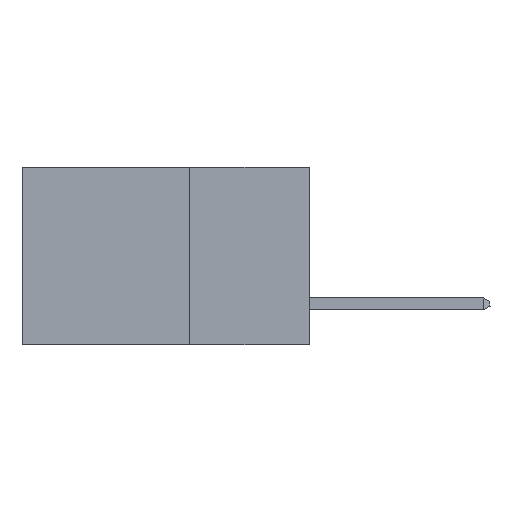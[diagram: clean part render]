
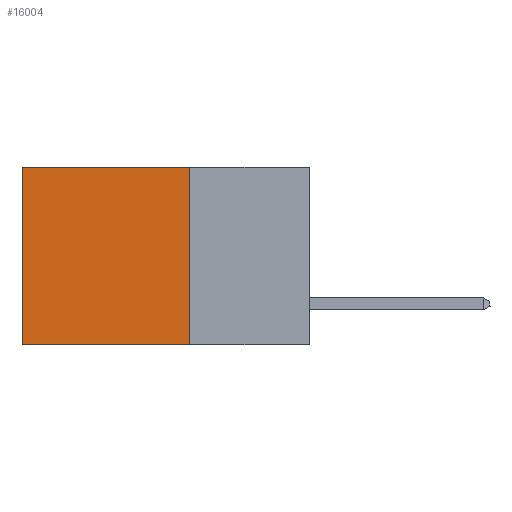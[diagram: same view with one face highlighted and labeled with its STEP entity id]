
A CAD part, left-side view. The second image highlights one B-rep face of the part: STEP entity #16004.
In plain terms, the highlighted planar face has unit normal (-1, 0, 0).
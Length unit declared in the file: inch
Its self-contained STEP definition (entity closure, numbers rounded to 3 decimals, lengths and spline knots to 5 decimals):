
#335 = VERTEX_POINT ( 'NONE', #10138 ) ;
#516 = LINE ( 'NONE', #1772, #23243 ) ;
#985 = EDGE_CURVE ( 'NONE', #22401, #9914, #516, .T. ) ;
#1112 = VECTOR ( 'NONE', #1794, 39.37008 ) ;
#1419 = CARTESIAN_POINT ( 'NONE',  ( 0.2875, 0.25, -0.37 ) ) ;
#1772 = CARTESIAN_POINT ( 'NONE',  ( 0.2875, 0.25, 0. ) ) ;
#1794 = DIRECTION ( 'NONE',  ( 0., 0., -1. ) ) ;
#2726 = CARTESIAN_POINT ( 'NONE',  ( 0.2875, 0.6, 0. ) ) ;
#3538 = CARTESIAN_POINT ( 'NONE',  ( 0.2875, 0.25, -0.37 ) ) ;
#4032 = LINE ( 'NONE', #3538, #8961 ) ;
#4887 = CARTESIAN_POINT ( 'NONE',  ( 0.2875, 0.6, 0. ) ) ;
#5421 = EDGE_CURVE ( 'NONE', #9914, #335, #20837, .T. ) ;
#6003 = DIRECTION ( 'NONE',  ( 1., 0., 0. ) ) ;
#8797 = ORIENTED_EDGE ( 'NONE', *, *, #13209, .F. ) ;
#8961 = VECTOR ( 'NONE', #10795, 39.37008 ) ;
#9129 = CARTESIAN_POINT ( 'NONE',  ( 0.2875, 0.25, 0. ) ) ;
#9348 = ORIENTED_EDGE ( 'NONE', *, *, #985, .T. ) ;
#9914 = VERTEX_POINT ( 'NONE', #4887 ) ;
#10138 = CARTESIAN_POINT ( 'NONE',  ( 0.2875, 0.6, -0.37 ) ) ;
#10795 = DIRECTION ( 'NONE',  ( 0., 1., 0. ) ) ;
#11484 = DIRECTION ( 'NONE',  ( 0., 1., 0. ) ) ;
#11539 = VECTOR ( 'NONE', #21451, 39.37008 ) ;
#11541 = EDGE_LOOP ( 'NONE', ( #13784, #11611, #8797, #9348 ) ) ;
#11611 = ORIENTED_EDGE ( 'NONE', *, *, #18734, .F. ) ;
#12321 = FACE_OUTER_BOUND ( 'NONE', #11541, .T. ) ;
#13209 = EDGE_CURVE ( 'NONE', #22401, #22803, #19763, .T. ) ;
#13784 = ORIENTED_EDGE ( 'NONE', *, *, #5421, .T. ) ;
#15054 = PLANE ( 'NONE',  #20317 ) ;
#16004 = ADVANCED_FACE ( 'NONE', ( #12321 ), #15054, .F. ) ;
#17102 = DIRECTION ( 'NONE',  ( 0., 0., -1. ) ) ;
#18734 = EDGE_CURVE ( 'NONE', #22803, #335, #4032, .T. ) ;
#19763 = LINE ( 'NONE', #20280, #1112 ) ;
#20280 = CARTESIAN_POINT ( 'NONE',  ( 0.2875, 0.25, 0. ) ) ;
#20317 = AXIS2_PLACEMENT_3D ( 'NONE', #22715, #6003, #17102 ) ;
#20837 = LINE ( 'NONE', #2726, #11539 ) ;
#21451 = DIRECTION ( 'NONE',  ( 0., 0., -1. ) ) ;
#22401 = VERTEX_POINT ( 'NONE', #9129 ) ;
#22715 = CARTESIAN_POINT ( 'NONE',  ( 0.2875, 0.25, 0. ) ) ;
#22803 = VERTEX_POINT ( 'NONE', #1419 ) ;
#23243 = VECTOR ( 'NONE', #11484, 39.37008 ) ;
